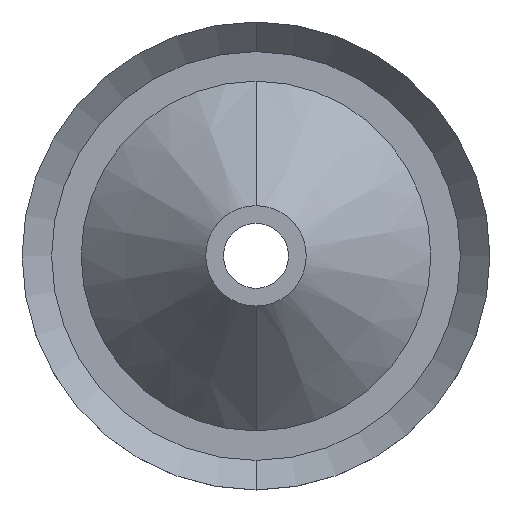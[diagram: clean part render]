
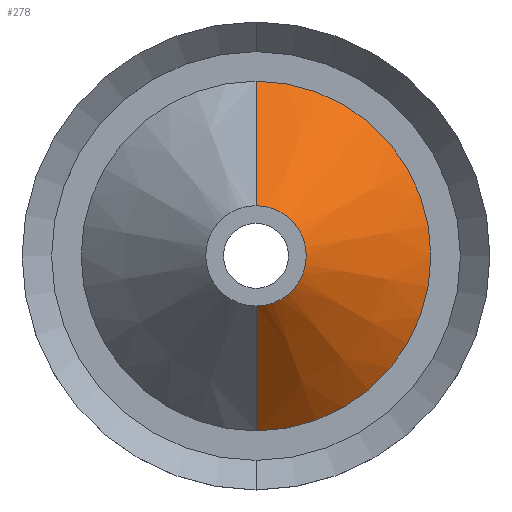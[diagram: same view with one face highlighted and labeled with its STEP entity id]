
A CAD part, top view. The second image highlights one B-rep face of the part: STEP entity #278.
In plain terms, the highlighted conical face has half-angle 45 degrees and reference radius 18.796 mm.
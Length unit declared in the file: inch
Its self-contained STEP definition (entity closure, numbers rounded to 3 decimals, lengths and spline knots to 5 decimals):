
#13 = AXIS2_PLACEMENT_3D ( 'NONE', #130, #187, #132 ) ;
#15 = DIRECTION ( 'NONE',  ( 0., 0., -1. ) ) ;
#22 = DIRECTION ( 'NONE',  ( 0., 1., 0. ) ) ;
#23 = ORIENTED_EDGE ( 'NONE', *, *, #577, .F. ) ;
#32 = VERTEX_POINT ( 'NONE', #505 ) ;
#82 = EDGE_LOOP ( 'NONE', ( #439, #195, #23, #506 ) ) ;
#121 = EDGE_CURVE ( 'NONE', #32, #180, #619, .T. ) ;
#130 = CARTESIAN_POINT ( 'NONE',  ( 0., 0., 0.7775 ) ) ;
#132 = DIRECTION ( 'NONE',  ( 0., 1., 0. ) ) ;
#140 = DIRECTION ( 'NONE',  ( 0., 0.707, -0.707 ) ) ;
#180 = VERTEX_POINT ( 'NONE', #569 ) ;
#187 = DIRECTION ( 'NONE',  ( 0., 0., -1. ) ) ;
#195 = ORIENTED_EDGE ( 'NONE', *, *, #645, .T. ) ;
#227 = CARTESIAN_POINT ( 'NONE',  ( 0., -0.2125, 0.7775 ) ) ;
#274 = DIRECTION ( 'NONE',  ( 0., 1., 0. ) ) ;
#278 = ADVANCED_FACE ( 'NONE', ( #315 ), #557, .T. ) ;
#286 = CARTESIAN_POINT ( 'NONE',  ( 0., 0., 0.25 ) ) ;
#315 = FACE_OUTER_BOUND ( 'NONE', #82, .T. ) ;
#340 = DIRECTION ( 'NONE',  ( 0., 0., -1. ) ) ;
#396 = AXIS2_PLACEMENT_3D ( 'NONE', #588, #15, #274 ) ;
#410 = CIRCLE ( 'NONE', #13, 0.2125 ) ;
#418 = CIRCLE ( 'NONE', #678, 0.74 ) ;
#439 = ORIENTED_EDGE ( 'NONE', *, *, #593, .T. ) ;
#442 = CARTESIAN_POINT ( 'NONE',  ( 0., -0.74, 0.25 ) ) ;
#501 = CARTESIAN_POINT ( 'NONE',  ( 0., -0.74, 0.25 ) ) ;
#505 = CARTESIAN_POINT ( 'NONE',  ( 0., 0.2125, 0.7775 ) ) ;
#506 = ORIENTED_EDGE ( 'NONE', *, *, #121, .F. ) ;
#508 = VERTEX_POINT ( 'NONE', #442 ) ;
#551 = VERTEX_POINT ( 'NONE', #227 ) ;
#553 = DIRECTION ( 'NONE',  ( 0., -0.707, -0.707 ) ) ;
#557 = CONICAL_SURFACE ( 'NONE', #396, 0.74, 0.785 ) ;
#569 = CARTESIAN_POINT ( 'NONE',  ( 0., 0.74, 0.25 ) ) ;
#577 = EDGE_CURVE ( 'NONE', #180, #508, #418, .T. ) ;
#588 = CARTESIAN_POINT ( 'NONE',  ( 0., 0., 0.25 ) ) ;
#593 = EDGE_CURVE ( 'NONE', #32, #551, #410, .T. ) ;
#619 = LINE ( 'NONE', #667, #669 ) ;
#645 = EDGE_CURVE ( 'NONE', #551, #508, #682, .T. ) ;
#667 = CARTESIAN_POINT ( 'NONE',  ( 0., 0.74, 0.25 ) ) ;
#668 = VECTOR ( 'NONE', #553, 39.37008 ) ;
#669 = VECTOR ( 'NONE', #140, 39.37008 ) ;
#678 = AXIS2_PLACEMENT_3D ( 'NONE', #286, #340, #22 ) ;
#682 = LINE ( 'NONE', #501, #668 ) ;
